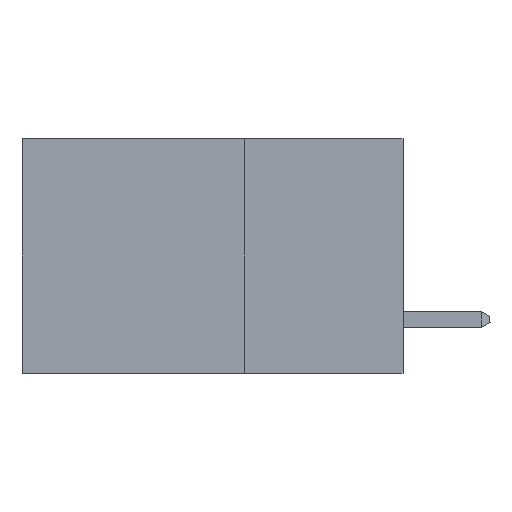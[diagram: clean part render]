
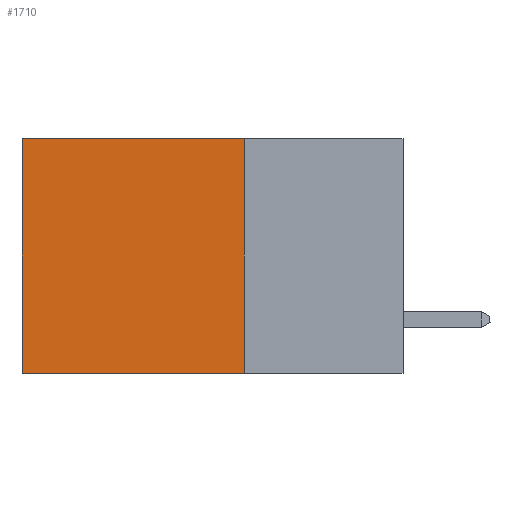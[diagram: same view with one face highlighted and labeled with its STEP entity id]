
A CAD part, left-side view. The second image highlights one B-rep face of the part: STEP entity #1710.
In plain terms, the highlighted planar face has unit normal (-1, 0, 0).
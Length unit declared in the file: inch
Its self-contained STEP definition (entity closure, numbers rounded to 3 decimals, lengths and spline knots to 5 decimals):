
#61 = DIRECTION ( 'NONE',  ( 0., 0., -1. ) ) ;
#144 = VECTOR ( 'NONE', #61, 39.37008 ) ;
#296 = LINE ( 'NONE', #6411, #5460 ) ;
#466 = DIRECTION ( 'NONE',  ( 1., 0., 0. ) ) ;
#1140 = DIRECTION ( 'NONE',  ( 0., 1., 0. ) ) ;
#1354 = VERTEX_POINT ( 'NONE', #2055 ) ;
#1655 = EDGE_CURVE ( 'NONE', #7549, #4617, #4265, .T. ) ;
#1710 = ADVANCED_FACE ( 'NONE', ( #6361 ), #8484, .F. ) ;
#2003 = LINE ( 'NONE', #8033, #7623 ) ;
#2055 = CARTESIAN_POINT ( 'NONE',  ( 0.2875, 0.6, -0.37 ) ) ;
#2882 = CARTESIAN_POINT ( 'NONE',  ( 0.2875, 0.6, 0. ) ) ;
#3101 = DIRECTION ( 'NONE',  ( 0., 0., -1. ) ) ;
#3158 = CARTESIAN_POINT ( 'NONE',  ( 0.2875, 0.25, 0. ) ) ;
#3220 = EDGE_CURVE ( 'NONE', #4797, #1354, #2003, .T. ) ;
#3608 = LINE ( 'NONE', #4162, #144 ) ;
#3788 = CARTESIAN_POINT ( 'NONE',  ( 0.2875, 0.25, 0. ) ) ;
#4162 = CARTESIAN_POINT ( 'NONE',  ( 0.2875, 0.6, 0. ) ) ;
#4247 = EDGE_CURVE ( 'NONE', #7549, #4797, #296, .T. ) ;
#4250 = VECTOR ( 'NONE', #1140, 39.37008 ) ;
#4265 = LINE ( 'NONE', #3158, #4250 ) ;
#4393 = ORIENTED_EDGE ( 'NONE', *, *, #6372, .T. ) ;
#4617 = VERTEX_POINT ( 'NONE', #2882 ) ;
#4635 = ORIENTED_EDGE ( 'NONE', *, *, #4247, .F. ) ;
#4797 = VERTEX_POINT ( 'NONE', #7172 ) ;
#5063 = AXIS2_PLACEMENT_3D ( 'NONE', #3788, #466, #3101 ) ;
#5319 = DIRECTION ( 'NONE',  ( 0., 1., 0. ) ) ;
#5460 = VECTOR ( 'NONE', #5725, 39.37008 ) ;
#5725 = DIRECTION ( 'NONE',  ( 0., 0., -1. ) ) ;
#5848 = ORIENTED_EDGE ( 'NONE', *, *, #1655, .T. ) ;
#5925 = ORIENTED_EDGE ( 'NONE', *, *, #3220, .F. ) ;
#6361 = FACE_OUTER_BOUND ( 'NONE', #8348, .T. ) ;
#6372 = EDGE_CURVE ( 'NONE', #4617, #1354, #3608, .T. ) ;
#6411 = CARTESIAN_POINT ( 'NONE',  ( 0.2875, 0.25, 0. ) ) ;
#7130 = CARTESIAN_POINT ( 'NONE',  ( 0.2875, 0.25, 0. ) ) ;
#7172 = CARTESIAN_POINT ( 'NONE',  ( 0.2875, 0.25, -0.37 ) ) ;
#7549 = VERTEX_POINT ( 'NONE', #7130 ) ;
#7623 = VECTOR ( 'NONE', #5319, 39.37008 ) ;
#8033 = CARTESIAN_POINT ( 'NONE',  ( 0.2875, 0.25, -0.37 ) ) ;
#8348 = EDGE_LOOP ( 'NONE', ( #4393, #5925, #4635, #5848 ) ) ;
#8484 = PLANE ( 'NONE',  #5063 ) ;
